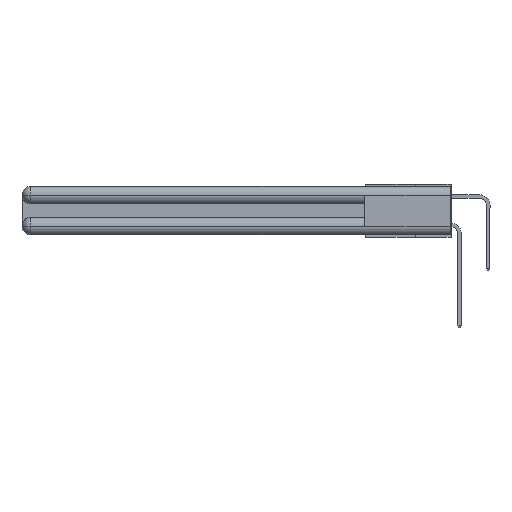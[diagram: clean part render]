
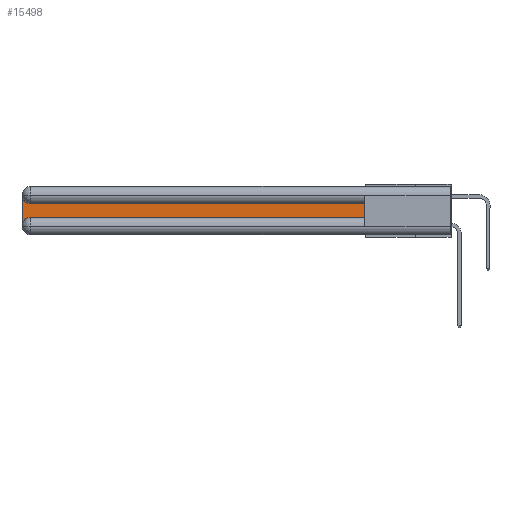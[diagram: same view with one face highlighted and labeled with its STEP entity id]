
A CAD part, left-side view. The second image highlights one B-rep face of the part: STEP entity #15498.
In plain terms, the highlighted planar face has unit normal (-1, 0, 0).
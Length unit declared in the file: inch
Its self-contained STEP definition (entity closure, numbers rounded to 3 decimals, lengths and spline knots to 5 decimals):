
#991 = DIRECTION ( 'NONE',  ( 0., 0., 1. ) ) ;
#1320 = VERTEX_POINT ( 'NONE', #18472 ) ;
#1715 = DIRECTION ( 'NONE',  ( 0., 0., -1. ) ) ;
#1814 = DIRECTION ( 'NONE',  ( 1., 0., 0. ) ) ;
#1986 = VECTOR ( 'NONE', #22979, 39.37008 ) ;
#2492 = EDGE_CURVE ( 'NONE', #3198, #25216, #10734, .T. ) ;
#3198 = VERTEX_POINT ( 'NONE', #4370 ) ;
#3606 = VERTEX_POINT ( 'NONE', #26638 ) ;
#3683 = DIRECTION ( 'NONE',  ( 0., 1., 0. ) ) ;
#4280 = CARTESIAN_POINT ( 'NONE',  ( 0.075, 0.6, -0.1225 ) ) ;
#4370 = CARTESIAN_POINT ( 'NONE',  ( 0.075, 0.6, -0.2175 ) ) ;
#4459 = DIRECTION ( 'NONE',  ( 0., 0., -1. ) ) ;
#5746 = CIRCLE ( 'NONE', #27274, 0.06 ) ;
#6082 = CARTESIAN_POINT ( 'NONE',  ( 0.075, 0.6, -0.1225 ) ) ;
#6367 = DIRECTION ( 'NONE',  ( 1., 0., 0. ) ) ;
#6461 = CARTESIAN_POINT ( 'NONE',  ( 0.075, 2.94, -0.0625 ) ) ;
#6748 = VECTOR ( 'NONE', #991, 39.37008 ) ;
#6918 = LINE ( 'NONE', #8527, #15856 ) ;
#6945 = LINE ( 'NONE', #6082, #7615 ) ;
#7587 = LINE ( 'NONE', #12689, #1986 ) ;
#7615 = VECTOR ( 'NONE', #3683, 39.37008 ) ;
#8491 = AXIS2_PLACEMENT_3D ( 'NONE', #6461, #21223, #23347 ) ;
#8527 = CARTESIAN_POINT ( 'NONE',  ( 0.075, 3., -0.2175 ) ) ;
#8605 = EDGE_CURVE ( 'NONE', #18501, #17038, #11303, .T. ) ;
#9123 = EDGE_CURVE ( 'NONE', #17038, #1320, #6918, .T. ) ;
#9303 = EDGE_CURVE ( 'NONE', #3606, #3198, #7587, .T. ) ;
#10068 = AXIS2_PLACEMENT_3D ( 'NONE', #25385, #6367, #21137 ) ;
#10081 = ORIENTED_EDGE ( 'NONE', *, *, #2492, .T. ) ;
#10507 = ORIENTED_EDGE ( 'NONE', *, *, #16020, .T. ) ;
#10635 = EDGE_LOOP ( 'NONE', ( #10507, #20623, #21252, #17015, #17254, #10081 ) ) ;
#10734 = LINE ( 'NONE', #15570, #6748 ) ;
#11303 = CIRCLE ( 'NONE', #8491, 0.06 ) ;
#12662 = EDGE_CURVE ( 'NONE', #1320, #3606, #5746, .T. ) ;
#12689 = CARTESIAN_POINT ( 'NONE',  ( 0.075, 0.6, -0.2175 ) ) ;
#14577 = CARTESIAN_POINT ( 'NONE',  ( 0.075, 2.94, -0.2775 ) ) ;
#15498 = ADVANCED_FACE ( 'NONE', ( #26461 ), #16910, .F. ) ;
#15570 = CARTESIAN_POINT ( 'NONE',  ( 0.075, 0.6, -0.2175 ) ) ;
#15856 = VECTOR ( 'NONE', #4459, 39.37008 ) ;
#16020 = EDGE_CURVE ( 'NONE', #25216, #18501, #6945, .T. ) ;
#16910 = PLANE ( 'NONE',  #10068 ) ;
#17015 = ORIENTED_EDGE ( 'NONE', *, *, #12662, .T. ) ;
#17038 = VERTEX_POINT ( 'NONE', #17391 ) ;
#17254 = ORIENTED_EDGE ( 'NONE', *, *, #9303, .T. ) ;
#17391 = CARTESIAN_POINT ( 'NONE',  ( 0.075, 3., -0.0625 ) ) ;
#18472 = CARTESIAN_POINT ( 'NONE',  ( 0.075, 3., -0.2775 ) ) ;
#18501 = VERTEX_POINT ( 'NONE', #20286 ) ;
#20286 = CARTESIAN_POINT ( 'NONE',  ( 0.075, 2.94, -0.1225 ) ) ;
#20623 = ORIENTED_EDGE ( 'NONE', *, *, #8605, .T. ) ;
#21137 = DIRECTION ( 'NONE',  ( 0., 0., -1. ) ) ;
#21223 = DIRECTION ( 'NONE',  ( 1., 0., 0. ) ) ;
#21252 = ORIENTED_EDGE ( 'NONE', *, *, #9123, .T. ) ;
#22979 = DIRECTION ( 'NONE',  ( 0., -1., 0. ) ) ;
#23347 = DIRECTION ( 'NONE',  ( 0., 0., -1. ) ) ;
#25216 = VERTEX_POINT ( 'NONE', #4280 ) ;
#25385 = CARTESIAN_POINT ( 'NONE',  ( 0.075, 3., -0.1225 ) ) ;
#26461 = FACE_OUTER_BOUND ( 'NONE', #10635, .T. ) ;
#26638 = CARTESIAN_POINT ( 'NONE',  ( 0.075, 2.94, -0.2175 ) ) ;
#27274 = AXIS2_PLACEMENT_3D ( 'NONE', #14577, #1814, #1715 ) ;
